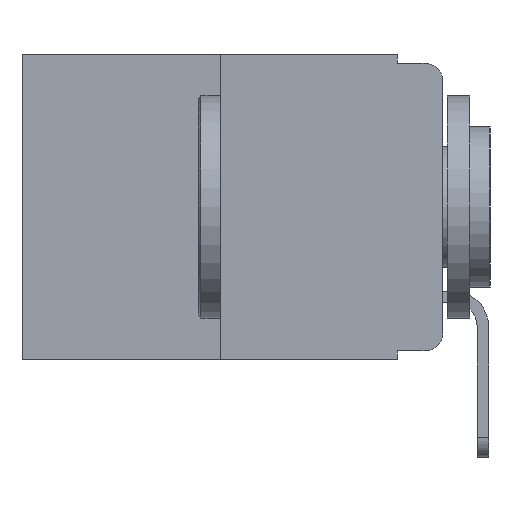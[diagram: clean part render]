
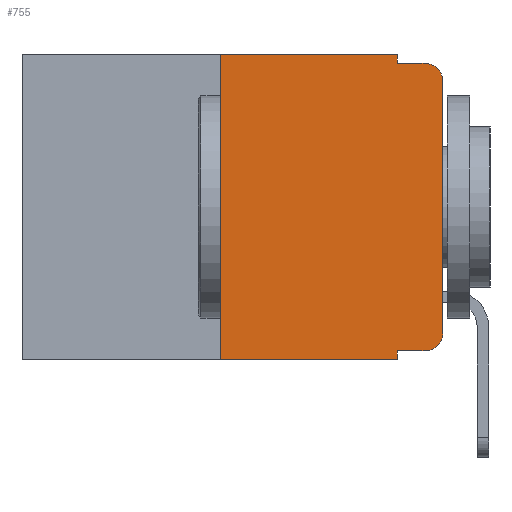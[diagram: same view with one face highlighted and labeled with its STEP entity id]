
A CAD part, left-side view. The second image highlights one B-rep face of the part: STEP entity #755.
In plain terms, the highlighted planar face has unit normal (-1, 0, 0).
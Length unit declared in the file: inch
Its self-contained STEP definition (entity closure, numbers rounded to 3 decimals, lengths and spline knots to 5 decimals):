
#104 = LINE ( 'NONE', #9315, #5426 ) ;
#384 = EDGE_CURVE ( 'NONE', #7697, #911, #10528, .T. ) ;
#442 = EDGE_CURVE ( 'NONE', #11542, #1325, #7603, .T. ) ;
#691 = EDGE_CURVE ( 'NONE', #8180, #5587, #6173, .T. ) ;
#755 = ADVANCED_FACE ( 'NONE', ( #3673 ), #1693, .F. ) ;
#911 = VERTEX_POINT ( 'NONE', #8634 ) ;
#1072 = DIRECTION ( 'NONE',  ( 0., 0., -1. ) ) ;
#1130 = AXIS2_PLACEMENT_3D ( 'NONE', #5568, #4910, #1072 ) ;
#1184 = DIRECTION ( 'NONE',  ( 0., -1., 0. ) ) ;
#1222 = VECTOR ( 'NONE', #3993, 39.37008 ) ;
#1325 = VERTEX_POINT ( 'NONE', #9557 ) ;
#1526 = CARTESIAN_POINT ( 'NONE',  ( 0., 0., 0. ) ) ;
#1590 = DIRECTION ( 'NONE',  ( 0., 0., 1. ) ) ;
#1693 = PLANE ( 'NONE',  #8567 ) ;
#1704 = DIRECTION ( 'NONE',  ( -1., 0., 0. ) ) ;
#1939 = ORIENTED_EDGE ( 'NONE', *, *, #9256, .F. ) ;
#1958 = VERTEX_POINT ( 'NONE', #9802 ) ;
#2012 = VECTOR ( 'NONE', #2026, 39.37008 ) ;
#2026 = DIRECTION ( 'NONE',  ( 0., -1., 0. ) ) ;
#2262 = ORIENTED_EDGE ( 'NONE', *, *, #5197, .T. ) ;
#2458 = CARTESIAN_POINT ( 'NONE',  ( 0., 0.473, -0.343 ) ) ;
#2461 = CARTESIAN_POINT ( 'NONE',  ( 0., 0.051, 0. ) ) ;
#2481 = CIRCLE ( 'NONE', #6606, 0.02 ) ;
#2561 = CARTESIAN_POINT ( 'NONE',  ( 0., 0., -0.03 ) ) ;
#2652 = CARTESIAN_POINT ( 'NONE',  ( 0., 0.25, -0.343 ) ) ;
#2815 = VECTOR ( 'NONE', #1184, 39.37008 ) ;
#2817 = DIRECTION ( 'NONE',  ( 0., 0., -1. ) ) ;
#2978 = VECTOR ( 'NONE', #10582, 39.37008 ) ;
#3418 = ORIENTED_EDGE ( 'NONE', *, *, #384, .F. ) ;
#3657 = CARTESIAN_POINT ( 'NONE',  ( 0., 0.02, -0.01 ) ) ;
#3673 = FACE_OUTER_BOUND ( 'NONE', #5101, .T. ) ;
#3711 = CARTESIAN_POINT ( 'NONE',  ( 0., 0.051, 0. ) ) ;
#3749 = CARTESIAN_POINT ( 'NONE',  ( 0., 0.02, -0.03 ) ) ;
#3993 = DIRECTION ( 'NONE',  ( 0., 0., -1. ) ) ;
#4052 = EDGE_CURVE ( 'NONE', #911, #1958, #5294, .T. ) ;
#4361 = DIRECTION ( 'NONE',  ( 0., 0., -1. ) ) ;
#4485 = DIRECTION ( 'NONE',  ( 0., 0., 1. ) ) ;
#4617 = LINE ( 'NONE', #3711, #1222 ) ;
#4910 = DIRECTION ( 'NONE',  ( -1., 0., 0. ) ) ;
#5101 = EDGE_LOOP ( 'NONE', ( #12214, #8137, #1939, #9252, #3418, #11023, #9619, #8463, #9809, #2262 ) ) ;
#5197 = EDGE_CURVE ( 'NONE', #1325, #9071, #10284, .T. ) ;
#5219 = CARTESIAN_POINT ( 'NONE',  ( 0., 0., -0.313 ) ) ;
#5280 = EDGE_CURVE ( 'NONE', #11542, #5587, #4617, .T. ) ;
#5294 = LINE ( 'NONE', #2461, #8103 ) ;
#5426 = VECTOR ( 'NONE', #9443, 39.37008 ) ;
#5439 = CARTESIAN_POINT ( 'NONE',  ( 0., 0.25, 0. ) ) ;
#5568 = CARTESIAN_POINT ( 'NONE',  ( 0., 0.02, -0.313 ) ) ;
#5587 = VERTEX_POINT ( 'NONE', #8390 ) ;
#6173 = LINE ( 'NONE', #2458, #2815 ) ;
#6488 = VERTEX_POINT ( 'NONE', #3657 ) ;
#6526 = CARTESIAN_POINT ( 'NONE',  ( 0., 0.051, -0.333 ) ) ;
#6547 = VERTEX_POINT ( 'NONE', #2561 ) ;
#6606 = AXIS2_PLACEMENT_3D ( 'NONE', #3749, #1704, #2817 ) ;
#7012 = EDGE_CURVE ( 'NONE', #8180, #7697, #12101, .T. ) ;
#7180 = LINE ( 'NONE', #1526, #9398 ) ;
#7470 = DIRECTION ( 'NONE',  ( 1., 0., 0. ) ) ;
#7560 = EDGE_CURVE ( 'NONE', #6547, #6488, #2481, .T. ) ;
#7603 = LINE ( 'NONE', #9526, #2012 ) ;
#7697 = VERTEX_POINT ( 'NONE', #9769 ) ;
#7727 = CARTESIAN_POINT ( 'NONE',  ( 0., 0.473, 0. ) ) ;
#8103 = VECTOR ( 'NONE', #4361, 39.37008 ) ;
#8137 = ORIENTED_EDGE ( 'NONE', *, *, #7560, .T. ) ;
#8180 = VERTEX_POINT ( 'NONE', #2652 ) ;
#8390 = CARTESIAN_POINT ( 'NONE',  ( 0., 0.051, -0.343 ) ) ;
#8463 = ORIENTED_EDGE ( 'NONE', *, *, #5280, .F. ) ;
#8567 = AXIS2_PLACEMENT_3D ( 'NONE', #10149, #7470, #10094 ) ;
#8634 = CARTESIAN_POINT ( 'NONE',  ( 0., 0.051, 0. ) ) ;
#8718 = EDGE_CURVE ( 'NONE', #9071, #6547, #7180, .T. ) ;
#9071 = VERTEX_POINT ( 'NONE', #5219 ) ;
#9252 = ORIENTED_EDGE ( 'NONE', *, *, #4052, .F. ) ;
#9256 = EDGE_CURVE ( 'NONE', #1958, #6488, #104, .T. ) ;
#9315 = CARTESIAN_POINT ( 'NONE',  ( 0., 0.051, -0.01 ) ) ;
#9398 = VECTOR ( 'NONE', #1590, 39.37008 ) ;
#9443 = DIRECTION ( 'NONE',  ( 0., -1., 0. ) ) ;
#9526 = CARTESIAN_POINT ( 'NONE',  ( 0., 0.051, -0.333 ) ) ;
#9557 = CARTESIAN_POINT ( 'NONE',  ( 0., 0.02, -0.333 ) ) ;
#9619 = ORIENTED_EDGE ( 'NONE', *, *, #691, .T. ) ;
#9769 = CARTESIAN_POINT ( 'NONE',  ( 0., 0.25, 0. ) ) ;
#9802 = CARTESIAN_POINT ( 'NONE',  ( 0., 0.051, -0.01 ) ) ;
#9809 = ORIENTED_EDGE ( 'NONE', *, *, #442, .T. ) ;
#10094 = DIRECTION ( 'NONE',  ( 0., 0., -1. ) ) ;
#10149 = CARTESIAN_POINT ( 'NONE',  ( 0., 0.473, 0. ) ) ;
#10284 = CIRCLE ( 'NONE', #1130, 0.02 ) ;
#10528 = LINE ( 'NONE', #7727, #2978 ) ;
#10582 = DIRECTION ( 'NONE',  ( 0., -1., 0. ) ) ;
#10590 = VECTOR ( 'NONE', #4485, 39.37008 ) ;
#11023 = ORIENTED_EDGE ( 'NONE', *, *, #7012, .F. ) ;
#11542 = VERTEX_POINT ( 'NONE', #6526 ) ;
#12101 = LINE ( 'NONE', #5439, #10590 ) ;
#12214 = ORIENTED_EDGE ( 'NONE', *, *, #8718, .T. ) ;
